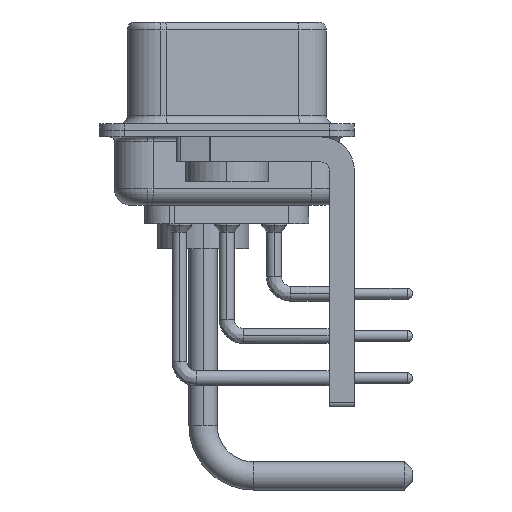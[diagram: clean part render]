
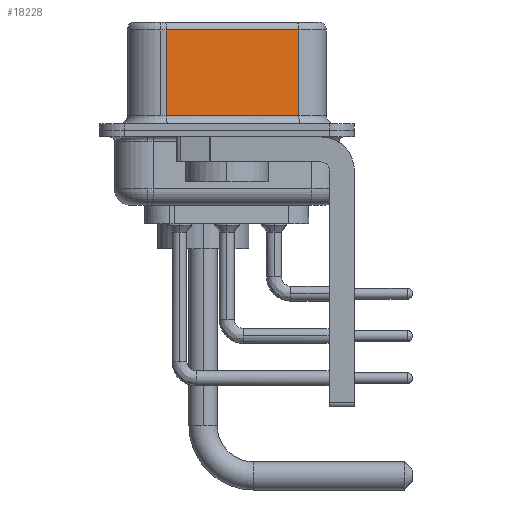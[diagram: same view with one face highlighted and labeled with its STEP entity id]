
A CAD part, left-side view. The second image highlights one B-rep face of the part: STEP entity #18228.
In plain terms, the highlighted planar face has unit normal (-0.985, -0.174, 0).
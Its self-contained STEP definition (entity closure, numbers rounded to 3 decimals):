
#634 = CARTESIAN_POINT ( 'NONE',  ( 5.132, -4.322, 0.9 ) ) ;
#2136 = VERTEX_POINT ( 'NONE', #19819 ) ;
#4493 = PLANE ( 'NONE',  #15315 ) ;
#6304 = VECTOR ( 'NONE', #8379, 1000. ) ;
#8379 = DIRECTION ( 'NONE',  ( -0.174, 0.985, 0. ) ) ;
#8978 = DIRECTION ( 'NONE',  ( 0.174, -0.985, 0. ) ) ;
#10346 = ORIENTED_EDGE ( 'NONE', *, *, #29334, .T. ) ;
#12636 = LINE ( 'NONE', #27177, #14457 ) ;
#12948 = EDGE_CURVE ( 'NONE', #2136, #25133, #12636, .T. ) ;
#13170 = CARTESIAN_POINT ( 'NONE',  ( 3.73, 3.628, 6.52 ) ) ;
#13196 = VECTOR ( 'NONE', #8978, 1000. ) ;
#13218 = CARTESIAN_POINT ( 'NONE',  ( 5.132, -4.322, 0.9 ) ) ;
#13233 = FACE_OUTER_BOUND ( 'NONE', #34309, .T. ) ;
#13419 = CARTESIAN_POINT ( 'NONE',  ( 5.132, -4.322, 6.52 ) ) ;
#14457 = VECTOR ( 'NONE', #30075, 1000. ) ;
#15315 = AXIS2_PLACEMENT_3D ( 'NONE', #13419, #36662, #19234 ) ;
#15960 = VECTOR ( 'NONE', #37169, 1000. ) ;
#16076 = ORIENTED_EDGE ( 'NONE', *, *, #30651, .T. ) ;
#17131 = LINE ( 'NONE', #32226, #6304 ) ;
#17923 = LINE ( 'NONE', #634, #13196 ) ;
#18228 = ADVANCED_FACE ( 'NONE', ( #13233 ), #4493, .F. ) ;
#18964 = CARTESIAN_POINT ( 'NONE',  ( 3.73, 3.628, 0.9 ) ) ;
#19234 = DIRECTION ( 'NONE',  ( -0.174, 0.985, 0. ) ) ;
#19819 = CARTESIAN_POINT ( 'NONE',  ( 5.132, -4.322, 6.02 ) ) ;
#24629 = VERTEX_POINT ( 'NONE', #36179 ) ;
#25133 = VERTEX_POINT ( 'NONE', #13218 ) ;
#25164 = LINE ( 'NONE', #13170, #15960 ) ;
#25572 = EDGE_CURVE ( 'NONE', #24629, #38168, #25164, .T. ) ;
#27177 = CARTESIAN_POINT ( 'NONE',  ( 5.132, -4.322, 6.52 ) ) ;
#28192 = ORIENTED_EDGE ( 'NONE', *, *, #12948, .F. ) ;
#29334 = EDGE_CURVE ( 'NONE', #2136, #24629, #17131, .T. ) ;
#30075 = DIRECTION ( 'NONE',  ( 0., 0., -1. ) ) ;
#30651 = EDGE_CURVE ( 'NONE', #38168, #25133, #17923, .T. ) ;
#32226 = CARTESIAN_POINT ( 'NONE',  ( 5.132, -4.322, 6.02 ) ) ;
#34309 = EDGE_LOOP ( 'NONE', ( #28192, #10346, #37521, #16076 ) ) ;
#36179 = CARTESIAN_POINT ( 'NONE',  ( 3.73, 3.628, 6.02 ) ) ;
#36662 = DIRECTION ( 'NONE',  ( 0.985, 0.174, 0. ) ) ;
#37169 = DIRECTION ( 'NONE',  ( 0., 0., -1. ) ) ;
#37521 = ORIENTED_EDGE ( 'NONE', *, *, #25572, .T. ) ;
#38168 = VERTEX_POINT ( 'NONE', #18964 ) ;
